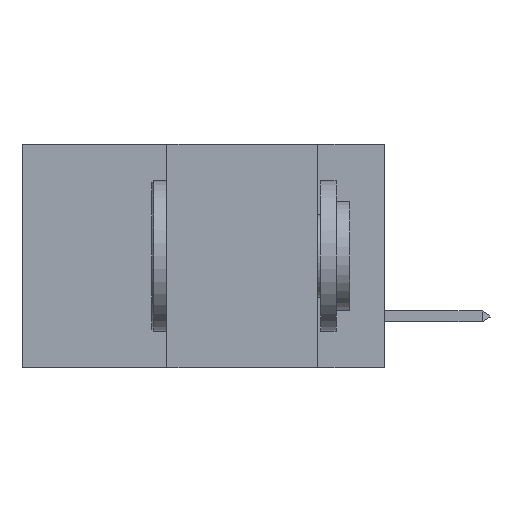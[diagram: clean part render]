
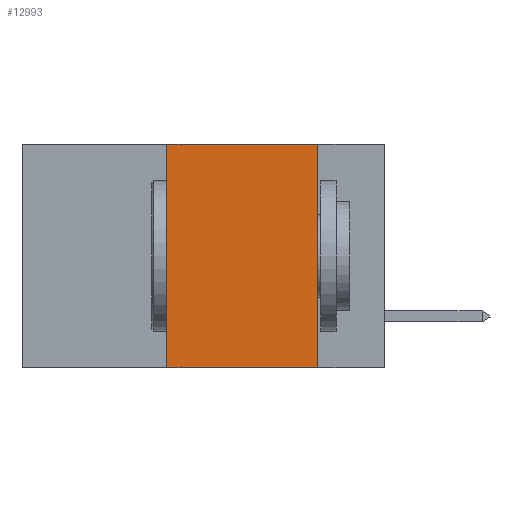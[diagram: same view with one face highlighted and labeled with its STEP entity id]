
A CAD part, left-side view. The second image highlights one B-rep face of the part: STEP entity #12993.
In plain terms, the highlighted planar face has unit normal (-1, 0, 0).
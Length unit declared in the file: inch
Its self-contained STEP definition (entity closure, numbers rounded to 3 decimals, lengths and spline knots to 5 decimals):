
#78 = DIRECTION ( 'NONE',  ( 0., 0., 1. ) ) ;
#300 = CARTESIAN_POINT ( 'NONE',  ( 0., 0.11, 0. ) ) ;
#342 = ORIENTED_EDGE ( 'NONE', *, *, #12867, .F. ) ;
#423 = CARTESIAN_POINT ( 'NONE',  ( 0., 0.6, 0. ) ) ;
#1063 = VECTOR ( 'NONE', #10231, 39.37008 ) ;
#1417 = LINE ( 'NONE', #6452, #10630 ) ;
#1541 = LINE ( 'NONE', #19280, #1063 ) ;
#3917 = CARTESIAN_POINT ( 'NONE',  ( 0., 0.6, -0.37 ) ) ;
#4341 = CARTESIAN_POINT ( 'NONE',  ( 0., 0.36, -0.37 ) ) ;
#4843 = DIRECTION ( 'NONE',  ( 1., 0., 0. ) ) ;
#5155 = LINE ( 'NONE', #3917, #17870 ) ;
#6452 = CARTESIAN_POINT ( 'NONE',  ( 0., 0.11, 0. ) ) ;
#6703 = ORIENTED_EDGE ( 'NONE', *, *, #8370, .F. ) ;
#7038 = DIRECTION ( 'NONE',  ( 0., -1., 0. ) ) ;
#7394 = FACE_OUTER_BOUND ( 'NONE', #15736, .T. ) ;
#7986 = CARTESIAN_POINT ( 'NONE',  ( 0., 0.11, -0.37 ) ) ;
#8370 = EDGE_CURVE ( 'NONE', #14336, #13111, #1417, .T. ) ;
#9596 = CARTESIAN_POINT ( 'NONE',  ( 0., 0.36, 0. ) ) ;
#9946 = EDGE_CURVE ( 'NONE', #16123, #13111, #5155, .T. ) ;
#10231 = DIRECTION ( 'NONE',  ( 0., -1., 0. ) ) ;
#10497 = CARTESIAN_POINT ( 'NONE',  ( 0., 0.36, 0. ) ) ;
#10630 = VECTOR ( 'NONE', #12357, 39.37008 ) ;
#12106 = LINE ( 'NONE', #10497, #16357 ) ;
#12357 = DIRECTION ( 'NONE',  ( 0., 0., -1. ) ) ;
#12775 = EDGE_CURVE ( 'NONE', #13774, #14336, #1541, .T. ) ;
#12867 = EDGE_CURVE ( 'NONE', #16123, #13774, #12106, .T. ) ;
#12993 = ADVANCED_FACE ( 'NONE', ( #7394 ), #15165, .F. ) ;
#13111 = VERTEX_POINT ( 'NONE', #7986 ) ;
#13774 = VERTEX_POINT ( 'NONE', #9596 ) ;
#14116 = ORIENTED_EDGE ( 'NONE', *, *, #12775, .F. ) ;
#14336 = VERTEX_POINT ( 'NONE', #300 ) ;
#14973 = ORIENTED_EDGE ( 'NONE', *, *, #9946, .T. ) ;
#15165 = PLANE ( 'NONE',  #17432 ) ;
#15736 = EDGE_LOOP ( 'NONE', ( #6703, #14116, #342, #14973 ) ) ;
#16123 = VERTEX_POINT ( 'NONE', #4341 ) ;
#16357 = VECTOR ( 'NONE', #78, 39.37008 ) ;
#16965 = DIRECTION ( 'NONE',  ( 0., 0., -1. ) ) ;
#17432 = AXIS2_PLACEMENT_3D ( 'NONE', #423, #4843, #16965 ) ;
#17870 = VECTOR ( 'NONE', #7038, 39.37008 ) ;
#19280 = CARTESIAN_POINT ( 'NONE',  ( 0., 0.6, 0. ) ) ;
